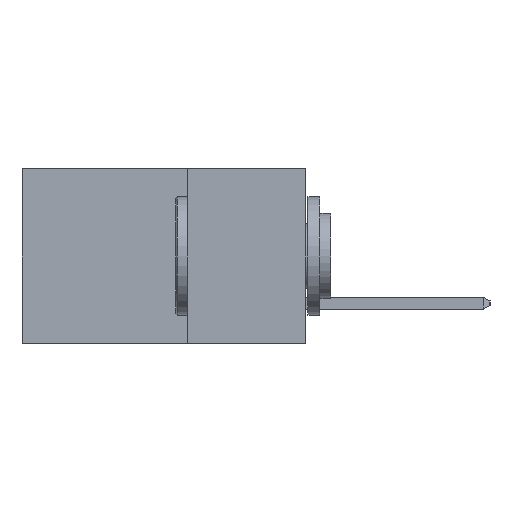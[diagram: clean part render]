
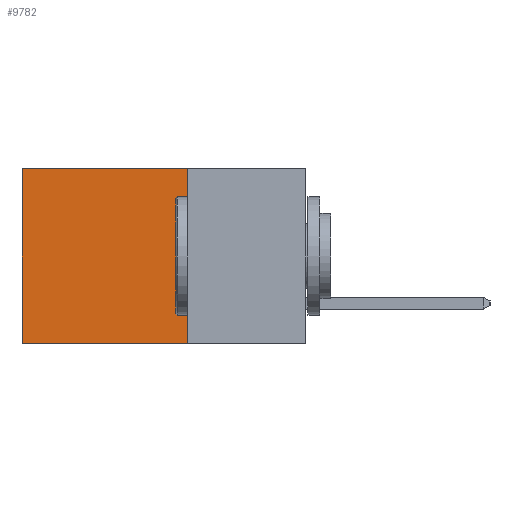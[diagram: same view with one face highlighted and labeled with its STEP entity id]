
A CAD part, left-side view. The second image highlights one B-rep face of the part: STEP entity #9782.
In plain terms, the highlighted planar face has unit normal (-1, 0, 0).
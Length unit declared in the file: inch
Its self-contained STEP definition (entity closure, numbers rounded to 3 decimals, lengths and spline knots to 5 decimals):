
#19 = EDGE_CURVE ( 'NONE', #16640, #16669, #13282, .T. ) ;
#299 = CARTESIAN_POINT ( 'NONE',  ( 0.2615, 0.25, -0.37 ) ) ;
#384 = DIRECTION ( 'NONE',  ( 0., 1., 0. ) ) ;
#511 = CARTESIAN_POINT ( 'NONE',  ( 0.2615, 0.25, 0. ) ) ;
#681 = VERTEX_POINT ( 'NONE', #17692 ) ;
#830 = ORIENTED_EDGE ( 'NONE', *, *, #5902, .F. ) ;
#1723 = VECTOR ( 'NONE', #11695, 39.37008 ) ;
#1867 = DIRECTION ( 'NONE',  ( 0., 0., -1. ) ) ;
#2116 = VECTOR ( 'NONE', #15862, 39.37008 ) ;
#4655 = EDGE_CURVE ( 'NONE', #681, #16669, #13660, .T. ) ;
#5902 = EDGE_CURVE ( 'NONE', #15239, #16640, #7289, .T. ) ;
#6313 = EDGE_LOOP ( 'NONE', ( #15433, #6900, #830, #6671 ) ) ;
#6449 = DIRECTION ( 'NONE',  ( 0., 0., -1. ) ) ;
#6453 = DIRECTION ( 'NONE',  ( 1., 0., 0. ) ) ;
#6473 = PLANE ( 'NONE',  #16730 ) ;
#6581 = CARTESIAN_POINT ( 'NONE',  ( 0.2615, 0.25, -0.37 ) ) ;
#6671 = ORIENTED_EDGE ( 'NONE', *, *, #10472, .T. ) ;
#6900 = ORIENTED_EDGE ( 'NONE', *, *, #19, .F. ) ;
#7075 = CARTESIAN_POINT ( 'NONE',  ( 0.2615, 0.25, -0.37 ) ) ;
#7289 = LINE ( 'NONE', #299, #14519 ) ;
#8312 = FACE_OUTER_BOUND ( 'NONE', #6313, .T. ) ;
#8599 = CARTESIAN_POINT ( 'NONE',  ( 0.2615, 0.6, -0.37 ) ) ;
#9782 = ADVANCED_FACE ( 'NONE', ( #8312 ), #6473, .F. ) ;
#10472 = EDGE_CURVE ( 'NONE', #15239, #681, #14362, .T. ) ;
#10533 = VECTOR ( 'NONE', #384, 39.37008 ) ;
#11695 = DIRECTION ( 'NONE',  ( 0., 1., 0. ) ) ;
#13282 = LINE ( 'NONE', #16855, #1723 ) ;
#13660 = LINE ( 'NONE', #15986, #2116 ) ;
#14362 = LINE ( 'NONE', #511, #10533 ) ;
#14519 = VECTOR ( 'NONE', #1867, 39.37008 ) ;
#15239 = VERTEX_POINT ( 'NONE', #15900 ) ;
#15433 = ORIENTED_EDGE ( 'NONE', *, *, #4655, .T. ) ;
#15862 = DIRECTION ( 'NONE',  ( 0., 0., -1. ) ) ;
#15900 = CARTESIAN_POINT ( 'NONE',  ( 0.2615, 0.25, 0. ) ) ;
#15986 = CARTESIAN_POINT ( 'NONE',  ( 0.2615, 0.6, -0.37 ) ) ;
#16640 = VERTEX_POINT ( 'NONE', #7075 ) ;
#16669 = VERTEX_POINT ( 'NONE', #8599 ) ;
#16730 = AXIS2_PLACEMENT_3D ( 'NONE', #6581, #6453, #6449 ) ;
#16855 = CARTESIAN_POINT ( 'NONE',  ( 0.2615, 0.25, -0.37 ) ) ;
#17692 = CARTESIAN_POINT ( 'NONE',  ( 0.2615, 0.6, 0. ) ) ;
